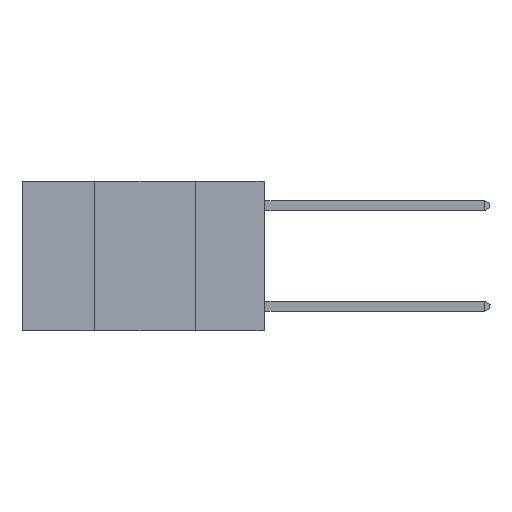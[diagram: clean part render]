
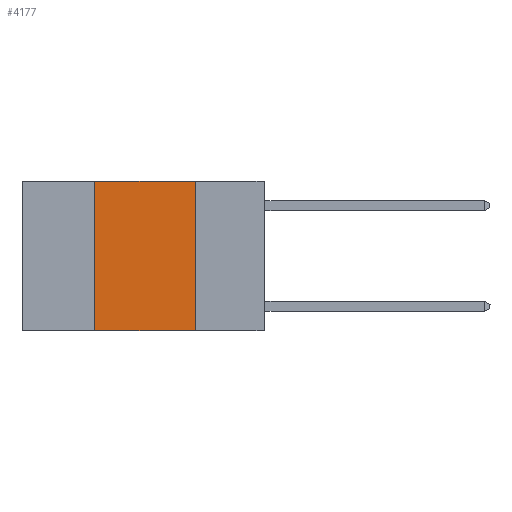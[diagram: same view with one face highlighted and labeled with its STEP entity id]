
A CAD part, left-side view. The second image highlights one B-rep face of the part: STEP entity #4177.
In plain terms, the highlighted planar face has unit normal (-1, 0, 0).
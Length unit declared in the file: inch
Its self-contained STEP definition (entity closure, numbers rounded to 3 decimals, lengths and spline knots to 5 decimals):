
#2342 = DIRECTION ( 'NONE',  ( 0., 0., 1. ) ) ;
#2476 = EDGE_LOOP ( 'NONE', ( #7125, #9434, #5447, #5701 ) ) ;
#2565 = PLANE ( 'NONE',  #3556 ) ;
#2781 = EDGE_CURVE ( 'NONE', #5357, #5043, #5236, .T. ) ;
#3556 = AXIS2_PLACEMENT_3D ( 'NONE', #9020, #4224, #9786 ) ;
#3557 = DIRECTION ( 'NONE',  ( 0., -1., 0. ) ) ;
#4177 = ADVANCED_FACE ( 'NONE', ( #7511 ), #2565, .F. ) ;
#4224 = DIRECTION ( 'NONE',  ( 1., 0., 0. ) ) ;
#4662 = VERTEX_POINT ( 'NONE', #10404 ) ;
#4826 = CARTESIAN_POINT ( 'NONE',  ( 0., 0.17, 0. ) ) ;
#4849 = LINE ( 'NONE', #5368, #6723 ) ;
#5043 = VERTEX_POINT ( 'NONE', #8532 ) ;
#5064 = EDGE_CURVE ( 'NONE', #4662, #5043, #4849, .T. ) ;
#5236 = LINE ( 'NONE', #6423, #9222 ) ;
#5357 = VERTEX_POINT ( 'NONE', #4826 ) ;
#5368 = CARTESIAN_POINT ( 'NONE',  ( 0., 0.6, -0.37 ) ) ;
#5447 = ORIENTED_EDGE ( 'NONE', *, *, #8357, .F. ) ;
#5449 = VECTOR ( 'NONE', #3557, 39.37008 ) ;
#5558 = CARTESIAN_POINT ( 'NONE',  ( 0., 0.42, 0. ) ) ;
#5616 = CARTESIAN_POINT ( 'NONE',  ( 0., 0.42, 0. ) ) ;
#5701 = ORIENTED_EDGE ( 'NONE', *, *, #5064, .T. ) ;
#5945 = VECTOR ( 'NONE', #2342, 39.37008 ) ;
#6027 = VERTEX_POINT ( 'NONE', #5616 ) ;
#6160 = DIRECTION ( 'NONE',  ( 0., -1., 0. ) ) ;
#6423 = CARTESIAN_POINT ( 'NONE',  ( 0., 0.17, 0. ) ) ;
#6723 = VECTOR ( 'NONE', #6160, 39.37008 ) ;
#7125 = ORIENTED_EDGE ( 'NONE', *, *, #2781, .F. ) ;
#7511 = FACE_OUTER_BOUND ( 'NONE', #2476, .T. ) ;
#7621 = LINE ( 'NONE', #9170, #5449 ) ;
#7957 = EDGE_CURVE ( 'NONE', #6027, #5357, #7621, .T. ) ;
#8115 = LINE ( 'NONE', #5558, #5945 ) ;
#8357 = EDGE_CURVE ( 'NONE', #4662, #6027, #8115, .T. ) ;
#8532 = CARTESIAN_POINT ( 'NONE',  ( 0., 0.17, -0.37 ) ) ;
#9020 = CARTESIAN_POINT ( 'NONE',  ( 0., 0.6, 0. ) ) ;
#9170 = CARTESIAN_POINT ( 'NONE',  ( 0., 0.6, 0. ) ) ;
#9222 = VECTOR ( 'NONE', #10465, 39.37008 ) ;
#9434 = ORIENTED_EDGE ( 'NONE', *, *, #7957, .F. ) ;
#9786 = DIRECTION ( 'NONE',  ( 0., 0., -1. ) ) ;
#10404 = CARTESIAN_POINT ( 'NONE',  ( 0., 0.42, -0.37 ) ) ;
#10465 = DIRECTION ( 'NONE',  ( 0., 0., -1. ) ) ;
